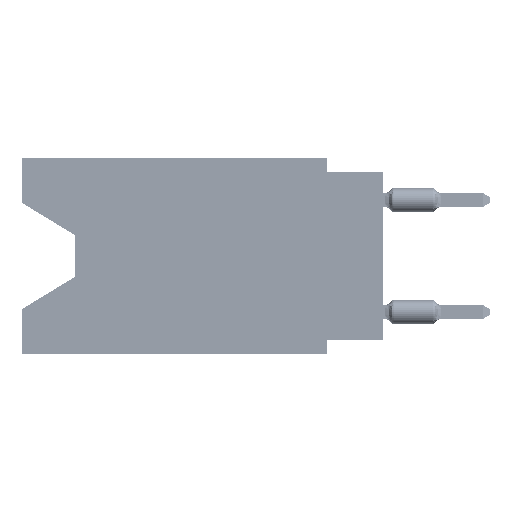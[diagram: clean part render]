
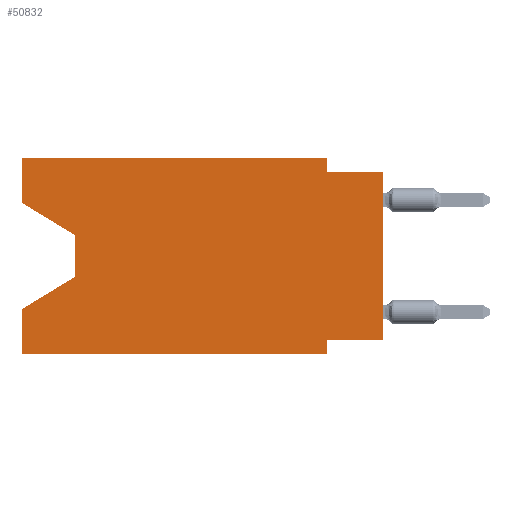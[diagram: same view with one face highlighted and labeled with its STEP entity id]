
A CAD part, left-side view. The second image highlights one B-rep face of the part: STEP entity #50832.
In plain terms, the highlighted planar face has unit normal (-1, 0, 0).
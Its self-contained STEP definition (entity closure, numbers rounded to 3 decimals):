
#2071 = EDGE_CURVE ( 'NONE', #45522, #99277, #31353, .T. ) ;
#4749 = PLANE ( 'NONE',  #36163 ) ;
#5367 = ORIENTED_EDGE ( 'NONE', *, *, #27467, .T. ) ;
#5738 = CARTESIAN_POINT ( 'NONE',  ( 0., 0., -0.635 ) ) ;
#6160 = VECTOR ( 'NONE', #9110, 1000. ) ;
#7167 = CARTESIAN_POINT ( 'NONE',  ( 0., 0., -0.635 ) ) ;
#8283 = EDGE_CURVE ( 'NONE', #110622, #45522, #106055, .T. ) ;
#9110 = DIRECTION ( 'NONE',  ( 0., 0., -1. ) ) ;
#10600 = VERTEX_POINT ( 'NONE', #88913 ) ;
#13404 = CARTESIAN_POINT ( 'NONE',  ( 0., 16.383, -8.89 ) ) ;
#14549 = ORIENTED_EDGE ( 'NONE', *, *, #54463, .F. ) ;
#14635 = DIRECTION ( 'NONE',  ( 1., 0., 0. ) ) ;
#14712 = ORIENTED_EDGE ( 'NONE', *, *, #88335, .T. ) ;
#15130 = DIRECTION ( 'NONE',  ( 0., 0.855, -0.519 ) ) ;
#15203 = VERTEX_POINT ( 'NONE', #95618 ) ;
#16421 = CARTESIAN_POINT ( 'NONE',  ( 0., 16.383, 0. ) ) ;
#16741 = EDGE_LOOP ( 'NONE', ( #38393, #105242, #14712, #77735, #5367, #66665, #27010, #108527, #14549, #80950, #62687, #25653 ) ) ;
#16807 = DIRECTION ( 'NONE',  ( 0., 0., 1. ) ) ;
#16972 = VECTOR ( 'NONE', #46037, 1000. ) ;
#17334 = VERTEX_POINT ( 'NONE', #7167 ) ;
#18385 = LINE ( 'NONE', #93730, #6160 ) ;
#21102 = VECTOR ( 'NONE', #76737, 1000. ) ;
#23012 = VECTOR ( 'NONE', #44816, 1000. ) ;
#23657 = EDGE_CURVE ( 'NONE', #101752, #75967, #63951, .T. ) ;
#25653 = ORIENTED_EDGE ( 'NONE', *, *, #23657, .F. ) ;
#27010 = ORIENTED_EDGE ( 'NONE', *, *, #8283, .F. ) ;
#27467 = EDGE_CURVE ( 'NONE', #105701, #99277, #43040, .T. ) ;
#28551 = LINE ( 'NONE', #55728, #120951 ) ;
#31353 = LINE ( 'NONE', #41214, #111331 ) ;
#36121 = LINE ( 'NONE', #110845, #116068 ) ;
#36163 = AXIS2_PLACEMENT_3D ( 'NONE', #70830, #14635, #61557 ) ;
#37966 = CARTESIAN_POINT ( 'NONE',  ( 0., 16.383, -2.038 ) ) ;
#38393 = ORIENTED_EDGE ( 'NONE', *, *, #120419, .T. ) ;
#40704 = CARTESIAN_POINT ( 'NONE',  ( 0., 16.383, -8.89 ) ) ;
#41214 = CARTESIAN_POINT ( 'NONE',  ( 0., 2.54, -8.89 ) ) ;
#42896 = CARTESIAN_POINT ( 'NONE',  ( 0., 16.383, 0. ) ) ;
#43040 = LINE ( 'NONE', #13404, #105615 ) ;
#44026 = LINE ( 'NONE', #5738, #47551 ) ;
#44501 = CARTESIAN_POINT ( 'NONE',  ( 0., 2.54, 0. ) ) ;
#44816 = DIRECTION ( 'NONE',  ( 0., 0., 1. ) ) ;
#45222 = LINE ( 'NONE', #82895, #71082 ) ;
#45522 = VERTEX_POINT ( 'NONE', #87920 ) ;
#46037 = DIRECTION ( 'NONE',  ( 0., -0.855, -0.519 ) ) ;
#47551 = VECTOR ( 'NONE', #73659, 1000. ) ;
#48320 = CARTESIAN_POINT ( 'NONE',  ( 0., 16.383, 0. ) ) ;
#50832 = ADVANCED_FACE ( 'NONE', ( #99246 ), #4749, .F. ) ;
#52107 = EDGE_CURVE ( 'NONE', #75967, #100338, #59160, .T. ) ;
#54463 = EDGE_CURVE ( 'NONE', #76804, #17334, #44026, .T. ) ;
#55728 = CARTESIAN_POINT ( 'NONE',  ( 0., 13.97, -3.505 ) ) ;
#56323 = DIRECTION ( 'NONE',  ( 0., 0., -1. ) ) ;
#56591 = CARTESIAN_POINT ( 'NONE',  ( 0., 13.97, -5.385 ) ) ;
#57418 = CARTESIAN_POINT ( 'NONE',  ( 0., 16.383, -2.038 ) ) ;
#59160 = LINE ( 'NONE', #85774, #114888 ) ;
#61557 = DIRECTION ( 'NONE',  ( 0., 0., -1. ) ) ;
#62687 = ORIENTED_EDGE ( 'NONE', *, *, #52107, .F. ) ;
#63951 = LINE ( 'NONE', #16421, #23012 ) ;
#66665 = ORIENTED_EDGE ( 'NONE', *, *, #2071, .F. ) ;
#67182 = EDGE_CURVE ( 'NONE', #110622, #17334, #45222, .T. ) ;
#68681 = LINE ( 'NONE', #48320, #21102 ) ;
#70830 = CARTESIAN_POINT ( 'NONE',  ( 0., 16.383, 0. ) ) ;
#71082 = VECTOR ( 'NONE', #16807, 1000. ) ;
#73659 = DIRECTION ( 'NONE',  ( 0., -1., 0. ) ) ;
#75967 = VERTEX_POINT ( 'NONE', #42896 ) ;
#76737 = DIRECTION ( 'NONE',  ( 0., 0., 1. ) ) ;
#76804 = VERTEX_POINT ( 'NONE', #91374 ) ;
#77112 = DIRECTION ( 'NONE',  ( 0., -1., 0. ) ) ;
#77735 = ORIENTED_EDGE ( 'NONE', *, *, #86699, .F. ) ;
#78898 = DIRECTION ( 'NONE',  ( 0., 0., -1. ) ) ;
#80950 = ORIENTED_EDGE ( 'NONE', *, *, #100851, .F. ) ;
#82895 = CARTESIAN_POINT ( 'NONE',  ( 0., 0., 0. ) ) ;
#85774 = CARTESIAN_POINT ( 'NONE',  ( 0., 16.383, 0. ) ) ;
#86699 = EDGE_CURVE ( 'NONE', #105701, #15203, #68681, .T. ) ;
#87529 = DIRECTION ( 'NONE',  ( 0., 1., 0. ) ) ;
#87920 = CARTESIAN_POINT ( 'NONE',  ( 0., 2.54, -8.255 ) ) ;
#88335 = EDGE_CURVE ( 'NONE', #111302, #15203, #36121, .T. ) ;
#88913 = CARTESIAN_POINT ( 'NONE',  ( 0., 13.97, -3.505 ) ) ;
#90577 = DIRECTION ( 'NONE',  ( 0., -1., 0. ) ) ;
#90703 = VECTOR ( 'NONE', #87529, 1000. ) ;
#91374 = CARTESIAN_POINT ( 'NONE',  ( 0., 2.54, -0.635 ) ) ;
#93730 = CARTESIAN_POINT ( 'NONE',  ( 0., 2.54, 0. ) ) ;
#95618 = CARTESIAN_POINT ( 'NONE',  ( 0., 16.383, -6.852 ) ) ;
#97401 = CARTESIAN_POINT ( 'NONE',  ( 0., 0., -8.255 ) ) ;
#98550 = CARTESIAN_POINT ( 'NONE',  ( 0., 2.54, -8.89 ) ) ;
#99246 = FACE_OUTER_BOUND ( 'NONE', #16741, .T. ) ;
#99277 = VERTEX_POINT ( 'NONE', #98550 ) ;
#100338 = VERTEX_POINT ( 'NONE', #44501 ) ;
#100851 = EDGE_CURVE ( 'NONE', #100338, #76804, #18385, .T. ) ;
#101752 = VERTEX_POINT ( 'NONE', #57418 ) ;
#105242 = ORIENTED_EDGE ( 'NONE', *, *, #105245, .T. ) ;
#105245 = EDGE_CURVE ( 'NONE', #10600, #111302, #28551, .T. ) ;
#105615 = VECTOR ( 'NONE', #90577, 1000. ) ;
#105701 = VERTEX_POINT ( 'NONE', #40704 ) ;
#106055 = LINE ( 'NONE', #97401, #90703 ) ;
#108527 = ORIENTED_EDGE ( 'NONE', *, *, #67182, .T. ) ;
#110622 = VERTEX_POINT ( 'NONE', #116760 ) ;
#110845 = CARTESIAN_POINT ( 'NONE',  ( 0., 13.97, -5.385 ) ) ;
#111302 = VERTEX_POINT ( 'NONE', #56591 ) ;
#111331 = VECTOR ( 'NONE', #78898, 1000. ) ;
#113318 = LINE ( 'NONE', #37966, #16972 ) ;
#114888 = VECTOR ( 'NONE', #77112, 1000. ) ;
#116068 = VECTOR ( 'NONE', #15130, 1000. ) ;
#116760 = CARTESIAN_POINT ( 'NONE',  ( 0., 0., -8.255 ) ) ;
#120419 = EDGE_CURVE ( 'NONE', #101752, #10600, #113318, .T. ) ;
#120951 = VECTOR ( 'NONE', #56323, 1000. ) ;
